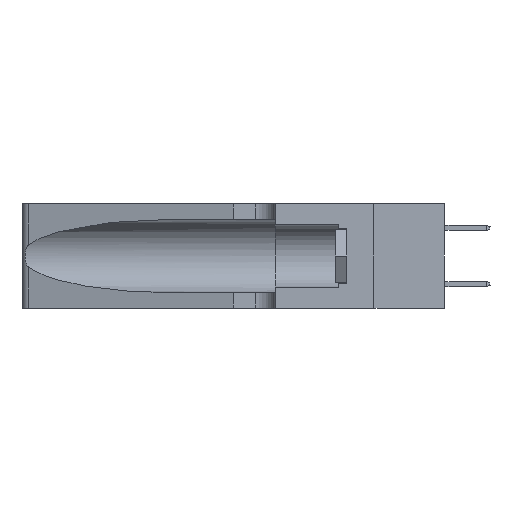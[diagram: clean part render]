
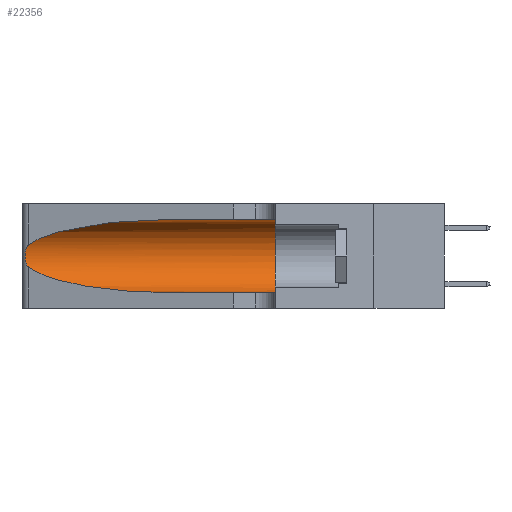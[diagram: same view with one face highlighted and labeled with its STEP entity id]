
A CAD part, left-side view. The second image highlights one B-rep face of the part: STEP entity #22356.
In plain terms, the highlighted cylindrical face has radius 3.308 mm (diameter 6.617 mm), a partial arc.
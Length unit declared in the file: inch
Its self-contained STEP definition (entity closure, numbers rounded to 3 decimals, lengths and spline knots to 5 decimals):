
#17 = CARTESIAN_POINT ( 'NONE',  ( 0.1305, 0.72297, 0.05475 ) ) ;
#656 = CARTESIAN_POINT ( 'NONE',  ( 0.25854, 1.2359, 0.20912 ) ) ;
#740 = DIRECTION ( 'NONE',  ( 0., -1., 0. ) ) ;
#1031 = CARTESIAN_POINT ( 'NONE',  ( 0.25487, 1.22718, 0.22369 ) ) ;
#1062 =( BOUNDED_CURVE ( )  B_SPLINE_CURVE ( 3, ( #7033, #3483, #10595, #17 ),
 .UNSPECIFIED., .F., .T. ) 
 B_SPLINE_CURVE_WITH_KNOTS ( ( 4, 4 ),
 ( 3.44316, 4.71239 ),
 .UNSPECIFIED. ) 
 CURVE ( )  GEOMETRIC_REPRESENTATION_ITEM ( )  RATIONAL_B_SPLINE_CURVE ( ( 1., 0.87, 0.87, 1. ) ) 
 REPRESENTATION_ITEM ( '' )  );
#1280 = VECTOR ( 'NONE', #7779, 39.37008 ) ;
#1694 = CARTESIAN_POINT ( 'NONE',  ( 0.25487, 1.22718, 0.22369 ) ) ;
#1872 = EDGE_CURVE ( 'NONE', #8608, #18361, #5126, .T. ) ;
#1890 = ORIENTED_EDGE ( 'NONE', *, *, #16620, .F. ) ;
#1954 = EDGE_LOOP ( 'NONE', ( #12062, #4374, #14798, #9094, #16320, #1890 ) ) ;
#2073 = CIRCLE ( 'NONE', #3563, 0.13025 ) ;
#2410 = CARTESIAN_POINT ( 'NONE',  ( 0.26075, 1.23896, 0.19203 ) ) ;
#3451 =( BOUNDED_CURVE ( )  B_SPLINE_CURVE ( 3, ( #8064, #22183, #11610, #1031 ),
 .UNSPECIFIED., .F., .T. ) 
 B_SPLINE_CURVE_WITH_KNOTS ( ( 4, 4 ),
 ( 1.5708, 2.84003 ),
 .UNSPECIFIED. ) 
 CURVE ( )  GEOMETRIC_REPRESENTATION_ITEM ( )  RATIONAL_B_SPLINE_CURVE ( ( 1., 0.87, 0.87, 1. ) ) 
 REPRESENTATION_ITEM ( '' )  );
#3483 = CARTESIAN_POINT ( 'NONE',  ( 0.2373, 1.15595, 0.08982 ) ) ;
#3563 = AXIS2_PLACEMENT_3D ( 'NONE', #7841, #20185, #9605 ) ;
#3584 = EDGE_CURVE ( 'NONE', #18361, #20666, #1062, .T. ) ;
#4169 = CARTESIAN_POINT ( 'NONE',  ( 0.26017, 1.23833, 0.17102 ) ) ;
#4374 = ORIENTED_EDGE ( 'NONE', *, *, #1872, .T. ) ;
#5126 = B_SPLINE_CURVE_WITH_KNOTS ( 'NONE', 3,
 ( #21796, #18231, #21721, #11227, #656, #12996, #2410, #14768, #4169, #16535, #5960, #18317, #7754, #20097 ),
 .UNSPECIFIED., .F., .F.,
 ( 4, 2, 2, 2, 2, 2, 4 ),
 ( 0., 0.00027, 0.00053, 0.00107, 0.0016, 0.00187, 0.00214 ),
 .UNSPECIFIED. ) ;
#5270 = VERTEX_POINT ( 'NONE', #19050 ) ;
#5570 = VERTEX_POINT ( 'NONE', #19803 ) ;
#5960 = CARTESIAN_POINT ( 'NONE',  ( 0.25789, 1.23486, 0.15765 ) ) ;
#7033 = CARTESIAN_POINT ( 'NONE',  ( 0.25487, 1.22718, 0.14631 ) ) ;
#7691 = CARTESIAN_POINT ( 'NONE',  ( 0.1305, 1.61858, 0.31525 ) ) ;
#7754 = CARTESIAN_POINT ( 'NONE',  ( 0.25555, 1.22993, 0.14849 ) ) ;
#7779 = DIRECTION ( 'NONE',  ( 0., -1., 0. ) ) ;
#7832 = FACE_OUTER_BOUND ( 'NONE', #1954, .T. ) ;
#7841 = CARTESIAN_POINT ( 'NONE',  ( 0.1305, 0.35, 0.185 ) ) ;
#8064 = CARTESIAN_POINT ( 'NONE',  ( 0.1305, 0.72297, 0.31525 ) ) ;
#8608 = VERTEX_POINT ( 'NONE', #1694 ) ;
#9053 = LINE ( 'NONE', #11316, #14312 ) ;
#9094 = ORIENTED_EDGE ( 'NONE', *, *, #12916, .T. ) ;
#9605 = DIRECTION ( 'NONE',  ( 0., 0., 1. ) ) ;
#9643 = CARTESIAN_POINT ( 'NONE',  ( 0.1305, 1.61858, 0.185 ) ) ;
#10544 = CARTESIAN_POINT ( 'NONE',  ( 0.1305, 0.72297, 0.05475 ) ) ;
#10595 = CARTESIAN_POINT ( 'NONE',  ( 0.18966, 0.96281, 0.05475 ) ) ;
#11227 = CARTESIAN_POINT ( 'NONE',  ( 0.25787, 1.23484, 0.2124 ) ) ;
#11316 = CARTESIAN_POINT ( 'NONE',  ( 0.1305, 1.61858, 0.05475 ) ) ;
#11610 = CARTESIAN_POINT ( 'NONE',  ( 0.2373, 1.15595, 0.28018 ) ) ;
#12011 = VERTEX_POINT ( 'NONE', #21281 ) ;
#12062 = ORIENTED_EDGE ( 'NONE', *, *, #13033, .T. ) ;
#12916 = EDGE_CURVE ( 'NONE', #20666, #5270, #9053, .T. ) ;
#12996 = CARTESIAN_POINT ( 'NONE',  ( 0.26018, 1.23835, 0.19895 ) ) ;
#13033 = EDGE_CURVE ( 'NONE', #12011, #8608, #3451, .T. ) ;
#13547 = AXIS2_PLACEMENT_3D ( 'NONE', #9643, #16644, #21989 ) ;
#14312 = VECTOR ( 'NONE', #740, 39.37008 ) ;
#14768 = CARTESIAN_POINT ( 'NONE',  ( 0.26075, 1.23896, 0.178 ) ) ;
#14798 = ORIENTED_EDGE ( 'NONE', *, *, #3584, .T. ) ;
#15905 = LINE ( 'NONE', #7691, #1280 ) ;
#16320 = ORIENTED_EDGE ( 'NONE', *, *, #17306, .F. ) ;
#16535 = CARTESIAN_POINT ( 'NONE',  ( 0.25856, 1.23593, 0.16098 ) ) ;
#16620 = EDGE_CURVE ( 'NONE', #12011, #5570, #15905, .T. ) ;
#16644 = DIRECTION ( 'NONE',  ( 0., -1., 0. ) ) ;
#17306 = EDGE_CURVE ( 'NONE', #5570, #5270, #2073, .T. ) ;
#18231 = CARTESIAN_POINT ( 'NONE',  ( 0.25555, 1.22994, 0.2215 ) ) ;
#18317 = CARTESIAN_POINT ( 'NONE',  ( 0.25639, 1.23186, 0.15144 ) ) ;
#18361 = VERTEX_POINT ( 'NONE', #22814 ) ;
#19050 = CARTESIAN_POINT ( 'NONE',  ( 0.1305, 0.35, 0.05475 ) ) ;
#19803 = CARTESIAN_POINT ( 'NONE',  ( 0.1305, 0.35, 0.31525 ) ) ;
#20097 = CARTESIAN_POINT ( 'NONE',  ( 0.25487, 1.22718, 0.14631 ) ) ;
#20185 = DIRECTION ( 'NONE',  ( 0., 1., 0. ) ) ;
#20666 = VERTEX_POINT ( 'NONE', #10544 ) ;
#21281 = CARTESIAN_POINT ( 'NONE',  ( 0.1305, 0.72297, 0.31525 ) ) ;
#21338 = CYLINDRICAL_SURFACE ( 'NONE', #13547, 0.13025 ) ;
#21721 = CARTESIAN_POINT ( 'NONE',  ( 0.25639, 1.23184, 0.21858 ) ) ;
#21796 = CARTESIAN_POINT ( 'NONE',  ( 0.25487, 1.22718, 0.22369 ) ) ;
#21989 = DIRECTION ( 'NONE',  ( 0., 0., -1. ) ) ;
#22183 = CARTESIAN_POINT ( 'NONE',  ( 0.18966, 0.96281, 0.31525 ) ) ;
#22356 = ADVANCED_FACE ( 'NONE', ( #7832 ), #21338, .F. ) ;
#22814 = CARTESIAN_POINT ( 'NONE',  ( 0.25487, 1.22718, 0.14631 ) ) ;
